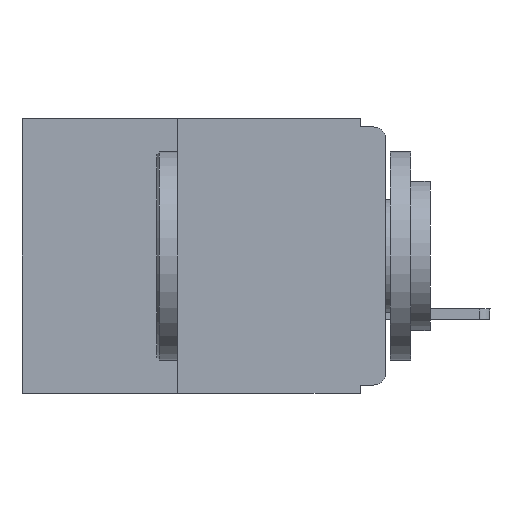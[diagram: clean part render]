
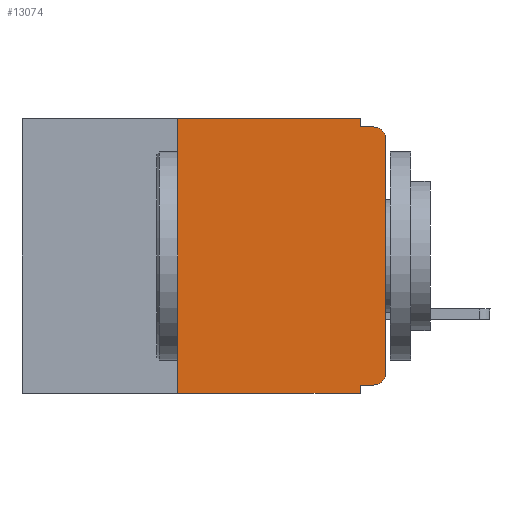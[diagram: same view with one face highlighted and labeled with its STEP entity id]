
A CAD part, left-side view. The second image highlights one B-rep face of the part: STEP entity #13074.
In plain terms, the highlighted planar face has unit normal (-1, 0, 0).
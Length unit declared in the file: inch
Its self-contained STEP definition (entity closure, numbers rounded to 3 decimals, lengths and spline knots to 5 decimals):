
#52 = CARTESIAN_POINT ( 'NONE',  ( 0., 0.031, 0. ) ) ;
#288 = CARTESIAN_POINT ( 'NONE',  ( 0., 0.437, 0. ) ) ;
#289 = ORIENTED_EDGE ( 'NONE', *, *, #10562, .T. ) ;
#453 = DIRECTION ( 'NONE',  ( 0., 0., -1. ) ) ;
#591 = LINE ( 'NONE', #2730, #14195 ) ;
#613 = CARTESIAN_POINT ( 'NONE',  ( 0., 0.437, -0.33 ) ) ;
#636 = EDGE_LOOP ( 'NONE', ( #7906, #289, #11164, #9224, #1202, #3749, #2100, #8566, #14400, #2061 ) ) ;
#637 = EDGE_CURVE ( 'NONE', #13478, #8445, #3310, .T. ) ;
#675 = CARTESIAN_POINT ( 'NONE',  ( 0., 0.015, -0.32 ) ) ;
#1089 = CARTESIAN_POINT ( 'NONE',  ( 0., 0.031, -0.32 ) ) ;
#1202 = ORIENTED_EDGE ( 'NONE', *, *, #9458, .F. ) ;
#1382 = LINE ( 'NONE', #8493, #13331 ) ;
#1428 = VERTEX_POINT ( 'NONE', #1089 ) ;
#1816 = DIRECTION ( 'NONE',  ( 0., -1., 0. ) ) ;
#1843 = CARTESIAN_POINT ( 'NONE',  ( 0., 0.031, -0.33 ) ) ;
#1914 = EDGE_CURVE ( 'NONE', #2815, #1428, #13951, .T. ) ;
#2036 = EDGE_CURVE ( 'NONE', #13478, #14655, #9610, .T. ) ;
#2061 = ORIENTED_EDGE ( 'NONE', *, *, #3698, .T. ) ;
#2100 = ORIENTED_EDGE ( 'NONE', *, *, #637, .T. ) ;
#2164 = CARTESIAN_POINT ( 'NONE',  ( 0., 0.25, 0. ) ) ;
#2178 = LINE ( 'NONE', #4821, #14330 ) ;
#2324 = EDGE_CURVE ( 'NONE', #1428, #8445, #8358, .T. ) ;
#2366 = VERTEX_POINT ( 'NONE', #12340 ) ;
#2394 = CARTESIAN_POINT ( 'NONE',  ( 0., 0.015, -0.01 ) ) ;
#2608 = PLANE ( 'NONE',  #11890 ) ;
#2730 = CARTESIAN_POINT ( 'NONE',  ( 0., 0., 0. ) ) ;
#2815 = VERTEX_POINT ( 'NONE', #675 ) ;
#2894 = VECTOR ( 'NONE', #14405, 39.37008 ) ;
#2895 = FACE_OUTER_BOUND ( 'NONE', #636, .T. ) ;
#3310 = LINE ( 'NONE', #613, #12359 ) ;
#3617 = DIRECTION ( 'NONE',  ( 0., -1., 0. ) ) ;
#3698 = EDGE_CURVE ( 'NONE', #2815, #3878, #14849, .T. ) ;
#3749 = ORIENTED_EDGE ( 'NONE', *, *, #2036, .F. ) ;
#3874 = VERTEX_POINT ( 'NONE', #2394 ) ;
#3878 = VERTEX_POINT ( 'NONE', #6942 ) ;
#4518 = DIRECTION ( 'NONE',  ( 0., 0., 1. ) ) ;
#4821 = CARTESIAN_POINT ( 'NONE',  ( 0., 0.437, 0. ) ) ;
#5042 = CARTESIAN_POINT ( 'NONE',  ( 0., 0.015, -0.025 ) ) ;
#5048 = VERTEX_POINT ( 'NONE', #52 ) ;
#5825 = EDGE_CURVE ( 'NONE', #5048, #2366, #1382, .T. ) ;
#6388 = CARTESIAN_POINT ( 'NONE',  ( 0., 0., -0.025 ) ) ;
#6622 = CARTESIAN_POINT ( 'NONE',  ( 0., 0.25, -0.33 ) ) ;
#6697 = VECTOR ( 'NONE', #453, 39.37008 ) ;
#6942 = CARTESIAN_POINT ( 'NONE',  ( 0., 0., -0.305 ) ) ;
#7051 = VECTOR ( 'NONE', #4518, 39.37008 ) ;
#7321 = DIRECTION ( 'NONE',  ( -1., 0., 0. ) ) ;
#7906 = ORIENTED_EDGE ( 'NONE', *, *, #11393, .T. ) ;
#8358 = LINE ( 'NONE', #8516, #6697 ) ;
#8363 = DIRECTION ( 'NONE',  ( 0., 0., 1. ) ) ;
#8445 = VERTEX_POINT ( 'NONE', #1843 ) ;
#8461 = LINE ( 'NONE', #9209, #10626 ) ;
#8493 = CARTESIAN_POINT ( 'NONE',  ( 0., 0.031, 0. ) ) ;
#8516 = CARTESIAN_POINT ( 'NONE',  ( 0., 0.031, -0.33 ) ) ;
#8566 = ORIENTED_EDGE ( 'NONE', *, *, #2324, .F. ) ;
#9209 = CARTESIAN_POINT ( 'NONE',  ( 0., 0., -0.01 ) ) ;
#9224 = ORIENTED_EDGE ( 'NONE', *, *, #5825, .F. ) ;
#9225 = CARTESIAN_POINT ( 'NONE',  ( 0., 0.25, -0.33 ) ) ;
#9458 = EDGE_CURVE ( 'NONE', #14655, #5048, #2178, .T. ) ;
#9610 = LINE ( 'NONE', #6622, #7051 ) ;
#9662 = DIRECTION ( 'NONE',  ( 0., 0., -1. ) ) ;
#10562 = EDGE_CURVE ( 'NONE', #10649, #3874, #13636, .T. ) ;
#10626 = VECTOR ( 'NONE', #14229, 39.37008 ) ;
#10649 = VERTEX_POINT ( 'NONE', #6388 ) ;
#11164 = ORIENTED_EDGE ( 'NONE', *, *, #14893, .F. ) ;
#11307 = AXIS2_PLACEMENT_3D ( 'NONE', #13591, #13495, #14520 ) ;
#11393 = EDGE_CURVE ( 'NONE', #3878, #10649, #591, .T. ) ;
#11601 = DIRECTION ( 'NONE',  ( 0., 0., -1. ) ) ;
#11890 = AXIS2_PLACEMENT_3D ( 'NONE', #288, #11911, #11601 ) ;
#11911 = DIRECTION ( 'NONE',  ( 1., 0., 0. ) ) ;
#12340 = CARTESIAN_POINT ( 'NONE',  ( 0., 0.031, -0.01 ) ) ;
#12359 = VECTOR ( 'NONE', #1816, 39.37008 ) ;
#13074 = ADVANCED_FACE ( 'NONE', ( #2895 ), #2608, .F. ) ;
#13215 = CARTESIAN_POINT ( 'NONE',  ( 0., 0., -0.32 ) ) ;
#13331 = VECTOR ( 'NONE', #14171, 39.37008 ) ;
#13478 = VERTEX_POINT ( 'NONE', #9225 ) ;
#13495 = DIRECTION ( 'NONE',  ( -1., 0., 0. ) ) ;
#13591 = CARTESIAN_POINT ( 'NONE',  ( 0., 0.015, -0.305 ) ) ;
#13636 = CIRCLE ( 'NONE', #14218, 0.015 ) ;
#13951 = LINE ( 'NONE', #13215, #2894 ) ;
#14171 = DIRECTION ( 'NONE',  ( 0., 0., -1. ) ) ;
#14195 = VECTOR ( 'NONE', #8363, 39.37008 ) ;
#14218 = AXIS2_PLACEMENT_3D ( 'NONE', #5042, #7321, #9662 ) ;
#14229 = DIRECTION ( 'NONE',  ( 0., -1., 0. ) ) ;
#14330 = VECTOR ( 'NONE', #3617, 39.37008 ) ;
#14400 = ORIENTED_EDGE ( 'NONE', *, *, #1914, .F. ) ;
#14405 = DIRECTION ( 'NONE',  ( 0., 1., 0. ) ) ;
#14520 = DIRECTION ( 'NONE',  ( 0., 0., -1. ) ) ;
#14655 = VERTEX_POINT ( 'NONE', #2164 ) ;
#14849 = CIRCLE ( 'NONE', #11307, 0.015 ) ;
#14893 = EDGE_CURVE ( 'NONE', #2366, #3874, #8461, .T. ) ;
